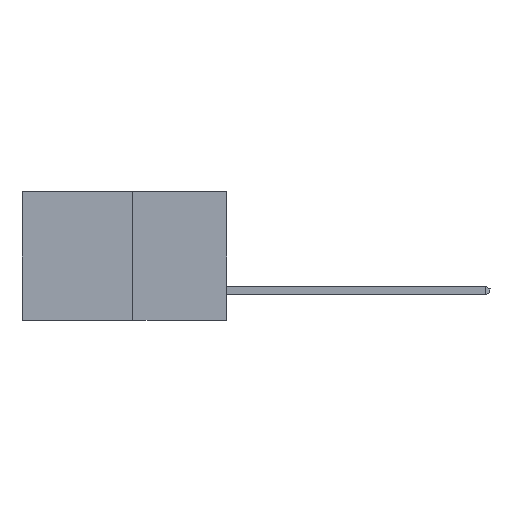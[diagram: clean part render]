
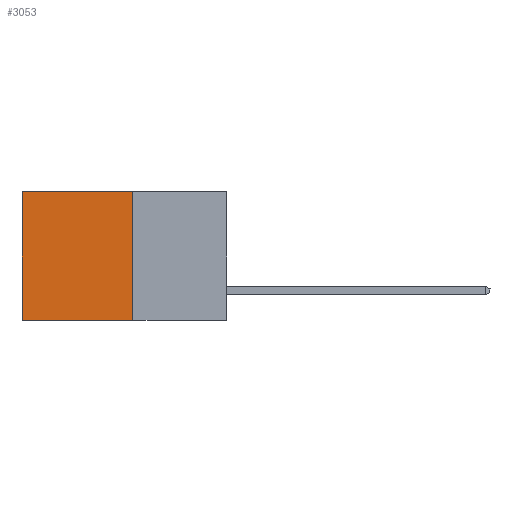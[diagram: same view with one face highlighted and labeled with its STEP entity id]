
A CAD part, left-side view. The second image highlights one B-rep face of the part: STEP entity #3053.
In plain terms, the highlighted planar face has unit normal (-1, 0, 0).
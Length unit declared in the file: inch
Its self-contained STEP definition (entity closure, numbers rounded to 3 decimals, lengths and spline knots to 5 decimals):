
#62 = VECTOR ( 'NONE', #8924, 39.37008 ) ;
#139 = CARTESIAN_POINT ( 'NONE',  ( 0.277, 0.27, -0.37 ) ) ;
#1969 = CARTESIAN_POINT ( 'NONE',  ( 0.277, 0.27, 0. ) ) ;
#2703 = CARTESIAN_POINT ( 'NONE',  ( 0.277, 0.27, -0.37 ) ) ;
#2720 = DIRECTION ( 'NONE',  ( 0., 1., 0. ) ) ;
#3053 = ADVANCED_FACE ( 'NONE', ( #9703 ), #8381, .F. ) ;
#3076 = VERTEX_POINT ( 'NONE', #7775 ) ;
#3500 = CARTESIAN_POINT ( 'NONE',  ( 0.277, 0.59, -0.37 ) ) ;
#3907 = EDGE_CURVE ( 'NONE', #5162, #7350, #11516, .T. ) ;
#4354 = AXIS2_PLACEMENT_3D ( 'NONE', #8571, #8318, #8301 ) ;
#4862 = CARTESIAN_POINT ( 'NONE',  ( 0.277, 0.27, -0.37 ) ) ;
#5162 = VERTEX_POINT ( 'NONE', #1969 ) ;
#5193 = ORIENTED_EDGE ( 'NONE', *, *, #6441, .F. ) ;
#6441 = EDGE_CURVE ( 'NONE', #7350, #10840, #10239, .T. ) ;
#7170 = LINE ( 'NONE', #9233, #12209 ) ;
#7350 = VERTEX_POINT ( 'NONE', #2703 ) ;
#7513 = EDGE_LOOP ( 'NONE', ( #12902, #5193, #7942, #13205 ) ) ;
#7518 = VECTOR ( 'NONE', #2720, 39.37008 ) ;
#7775 = CARTESIAN_POINT ( 'NONE',  ( 0.277, 0.59, 0. ) ) ;
#7942 = ORIENTED_EDGE ( 'NONE', *, *, #3907, .F. ) ;
#8301 = DIRECTION ( 'NONE',  ( 0., 0., -1. ) ) ;
#8318 = DIRECTION ( 'NONE',  ( 1., 0., 0. ) ) ;
#8381 = PLANE ( 'NONE',  #4354 ) ;
#8571 = CARTESIAN_POINT ( 'NONE',  ( 0.277, 0.27, -0.37 ) ) ;
#8711 = EDGE_CURVE ( 'NONE', #3076, #10840, #12607, .T. ) ;
#8924 = DIRECTION ( 'NONE',  ( 0., 0., -1. ) ) ;
#9233 = CARTESIAN_POINT ( 'NONE',  ( 0.277, 0.27, 0. ) ) ;
#9703 = FACE_OUTER_BOUND ( 'NONE', #7513, .T. ) ;
#10021 = VECTOR ( 'NONE', #12712, 39.37008 ) ;
#10214 = DIRECTION ( 'NONE',  ( 0., 1., 0. ) ) ;
#10239 = LINE ( 'NONE', #4862, #7518 ) ;
#10271 = CARTESIAN_POINT ( 'NONE',  ( 0.277, 0.59, -0.37 ) ) ;
#10840 = VERTEX_POINT ( 'NONE', #10271 ) ;
#11516 = LINE ( 'NONE', #139, #62 ) ;
#11617 = EDGE_CURVE ( 'NONE', #5162, #3076, #7170, .T. ) ;
#12209 = VECTOR ( 'NONE', #10214, 39.37008 ) ;
#12607 = LINE ( 'NONE', #3500, #10021 ) ;
#12712 = DIRECTION ( 'NONE',  ( 0., 0., -1. ) ) ;
#12902 = ORIENTED_EDGE ( 'NONE', *, *, #8711, .T. ) ;
#13205 = ORIENTED_EDGE ( 'NONE', *, *, #11617, .T. ) ;
